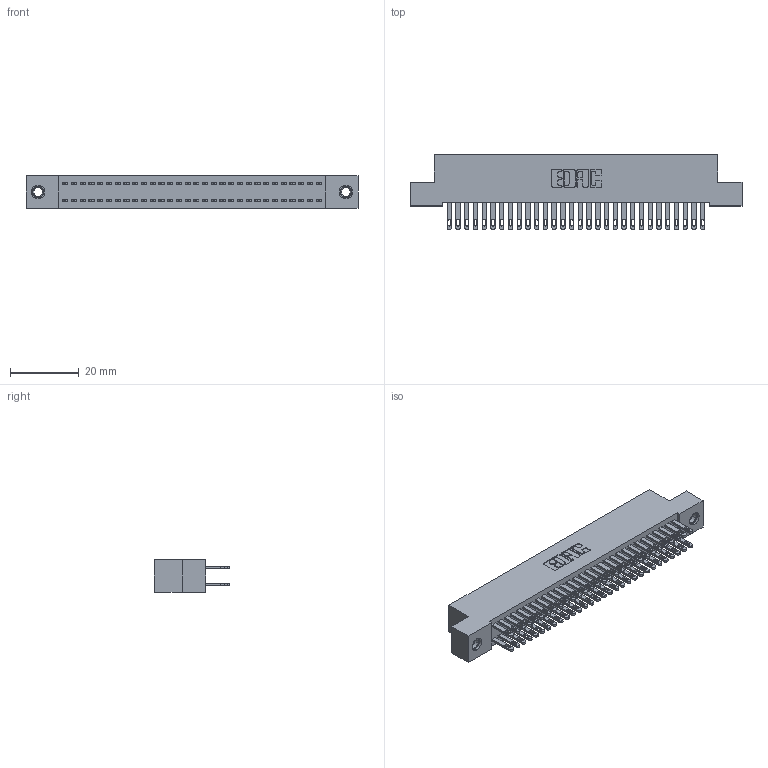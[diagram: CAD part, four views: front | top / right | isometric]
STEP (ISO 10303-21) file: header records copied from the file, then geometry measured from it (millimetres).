
FILE_DESCRIPTION (( 'STEP AP203' ), '1' );
FILE_NAME ('892-060-500-207.STEP', '2020-09-21T19:10:19', ( '' ), ( '' ), 'SwSTEP 2.0', 'SolidWorks 2020', '' );
FILE_SCHEMA (( 'CONFIG_CONTROL_DESIGN' ));
Length unit declared in the file: inch
Products named in the file (4): 892-060-500-207; 345-250-001_345-250-005-103; 345-292-001_345-293-100; 842 Part_TI
Assembly tree (63 placements, depth 2):
  892-060-500-207
    842 Part_TI
    345-292-001_345-293-100  x60
    345-250-001_345-250-005-103  x2
Bounding box: 96.52 x 21.85 x 9.4 mm (x, y, z)
Volume: 8786.2 mm3; surface area: 14606.2 mm2
Topology: 63 solids, 63 shells, 3050 faces, 9255 edges, 6162 vertices
Faces by surface type: plane 1898, cylinder 1136, cone 12, torus 4
Entity records: 21836 total; most frequent: CARTESIAN_POINT 3613, ORIENTED_EDGE 3542, DIRECTION 3141, EDGE_CURVE 1771, VECTOR 1619, LINE 1619, VERTEX_POINT 1176, AXIS2_PLACEMENT_3D 761
